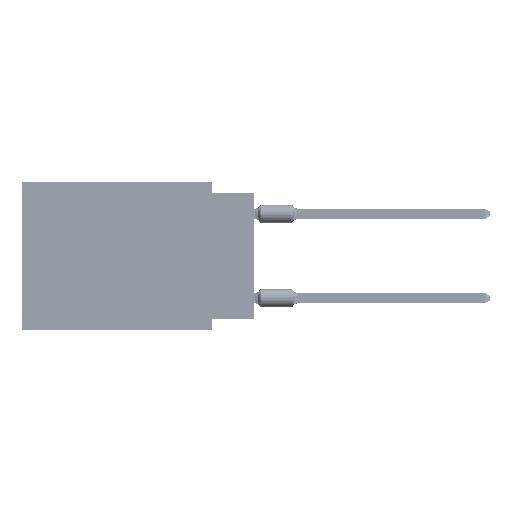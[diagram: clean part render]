
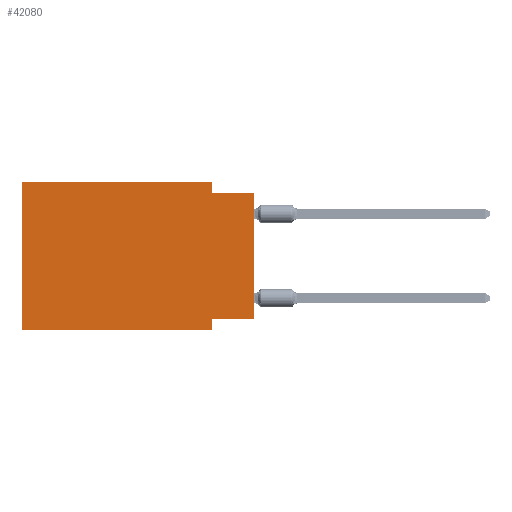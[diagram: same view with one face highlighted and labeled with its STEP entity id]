
A CAD part, left-side view. The second image highlights one B-rep face of the part: STEP entity #42080.
In plain terms, the highlighted planar face has unit normal (-1, 0, 0).
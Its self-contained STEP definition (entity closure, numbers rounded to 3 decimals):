
#1222 = DIRECTION ( 'NONE',  ( 1., 0., 0. ) ) ;
#2618 = CARTESIAN_POINT ( 'NONE',  ( 0., 13.97, 0. ) ) ;
#6146 = ORIENTED_EDGE ( 'NONE', *, *, #37566, .F. ) ;
#8743 = DIRECTION ( 'NONE',  ( 0., 1., 0. ) ) ;
#9361 = LINE ( 'NONE', #73215, #101247 ) ;
#9810 = DIRECTION ( 'NONE',  ( 0., -1., 0. ) ) ;
#12685 = VECTOR ( 'NONE', #8743, 1000. ) ;
#17072 = DIRECTION ( 'NONE',  ( 0., 0., -1. ) ) ;
#21448 = CARTESIAN_POINT ( 'NONE',  ( 0., 2.54, -8.255 ) ) ;
#21904 = ORIENTED_EDGE ( 'NONE', *, *, #73822, .T. ) ;
#23025 = VECTOR ( 'NONE', #17072, 1000. ) ;
#26435 = CARTESIAN_POINT ( 'NONE',  ( 0., 13.97, -8.89 ) ) ;
#26450 = EDGE_CURVE ( 'NONE', #58128, #40109, #83296, .T. ) ;
#28181 = DIRECTION ( 'NONE',  ( 0., 0., 1. ) ) ;
#30220 = DIRECTION ( 'NONE',  ( 0., 0., -1. ) ) ;
#31673 = VERTEX_POINT ( 'NONE', #73737 ) ;
#34954 = LINE ( 'NONE', #26435, #72234 ) ;
#37566 = EDGE_CURVE ( 'NONE', #31673, #114627, #83166, .T. ) ;
#38385 = VERTEX_POINT ( 'NONE', #62827 ) ;
#40109 = VERTEX_POINT ( 'NONE', #110147 ) ;
#41748 = CARTESIAN_POINT ( 'NONE',  ( 0., 2.54, 0. ) ) ;
#42080 = ADVANCED_FACE ( 'NONE', ( #75355 ), #84486, .F. ) ;
#44397 = CARTESIAN_POINT ( 'NONE',  ( 0., 2.54, -8.89 ) ) ;
#44657 = DIRECTION ( 'NONE',  ( 0., -1., 0. ) ) ;
#47488 = VERTEX_POINT ( 'NONE', #95108 ) ;
#47973 = CARTESIAN_POINT ( 'NONE',  ( 0., 13.97, 0. ) ) ;
#48458 = CARTESIAN_POINT ( 'NONE',  ( 0., 2.54, 0. ) ) ;
#48533 = EDGE_CURVE ( 'NONE', #49252, #38385, #9361, .T. ) ;
#49252 = VERTEX_POINT ( 'NONE', #115574 ) ;
#50144 = ORIENTED_EDGE ( 'NONE', *, *, #81148, .F. ) ;
#50477 = VECTOR ( 'NONE', #113276, 1000. ) ;
#51830 = ORIENTED_EDGE ( 'NONE', *, *, #77351, .F. ) ;
#53584 = ORIENTED_EDGE ( 'NONE', *, *, #48533, .T. ) ;
#57202 = CARTESIAN_POINT ( 'NONE',  ( 0., 0., -0.635 ) ) ;
#57311 = LINE ( 'NONE', #2618, #50477 ) ;
#58128 = VERTEX_POINT ( 'NONE', #21448 ) ;
#58265 = VERTEX_POINT ( 'NONE', #62741 ) ;
#59818 = VECTOR ( 'NONE', #71037, 1000. ) ;
#62741 = CARTESIAN_POINT ( 'NONE',  ( 0., 13.97, -8.89 ) ) ;
#62827 = CARTESIAN_POINT ( 'NONE',  ( 0., 0., -0.635 ) ) ;
#70329 = ORIENTED_EDGE ( 'NONE', *, *, #26450, .F. ) ;
#71037 = DIRECTION ( 'NONE',  ( 0., -1., 0. ) ) ;
#71444 = VECTOR ( 'NONE', #30220, 1000. ) ;
#72234 = VECTOR ( 'NONE', #44657, 1000. ) ;
#73215 = CARTESIAN_POINT ( 'NONE',  ( 0., 0., 0. ) ) ;
#73737 = CARTESIAN_POINT ( 'NONE',  ( 0., 13.97, 0. ) ) ;
#73822 = EDGE_CURVE ( 'NONE', #58265, #40109, #34954, .T. ) ;
#75355 = FACE_OUTER_BOUND ( 'NONE', #82578, .T. ) ;
#75428 = ORIENTED_EDGE ( 'NONE', *, *, #106738, .F. ) ;
#77351 = EDGE_CURVE ( 'NONE', #49252, #58128, #92035, .T. ) ;
#78548 = CARTESIAN_POINT ( 'NONE',  ( 0., 13.97, 0. ) ) ;
#81148 = EDGE_CURVE ( 'NONE', #114627, #47488, #113555, .T. ) ;
#81688 = CARTESIAN_POINT ( 'NONE',  ( 0., 0., -8.255 ) ) ;
#82578 = EDGE_LOOP ( 'NONE', ( #53584, #75428, #50144, #6146, #100927, #21904, #70329, #51830 ) ) ;
#83166 = LINE ( 'NONE', #78548, #59818 ) ;
#83296 = LINE ( 'NONE', #44397, #23025 ) ;
#84486 = PLANE ( 'NONE',  #113751 ) ;
#88592 = VECTOR ( 'NONE', #9810, 1000. ) ;
#92035 = LINE ( 'NONE', #81688, #12685 ) ;
#95108 = CARTESIAN_POINT ( 'NONE',  ( 0., 2.54, -0.635 ) ) ;
#100927 = ORIENTED_EDGE ( 'NONE', *, *, #110170, .F. ) ;
#101247 = VECTOR ( 'NONE', #28181, 1000. ) ;
#106738 = EDGE_CURVE ( 'NONE', #47488, #38385, #110753, .T. ) ;
#110147 = CARTESIAN_POINT ( 'NONE',  ( 0., 2.54, -8.89 ) ) ;
#110170 = EDGE_CURVE ( 'NONE', #58265, #31673, #57311, .T. ) ;
#110753 = LINE ( 'NONE', #57202, #88592 ) ;
#113276 = DIRECTION ( 'NONE',  ( 0., 0., 1. ) ) ;
#113555 = LINE ( 'NONE', #48458, #71444 ) ;
#113751 = AXIS2_PLACEMENT_3D ( 'NONE', #47973, #1222, #114844 ) ;
#114627 = VERTEX_POINT ( 'NONE', #41748 ) ;
#114844 = DIRECTION ( 'NONE',  ( 0., 0., -1. ) ) ;
#115574 = CARTESIAN_POINT ( 'NONE',  ( 0., 0., -8.255 ) ) ;
